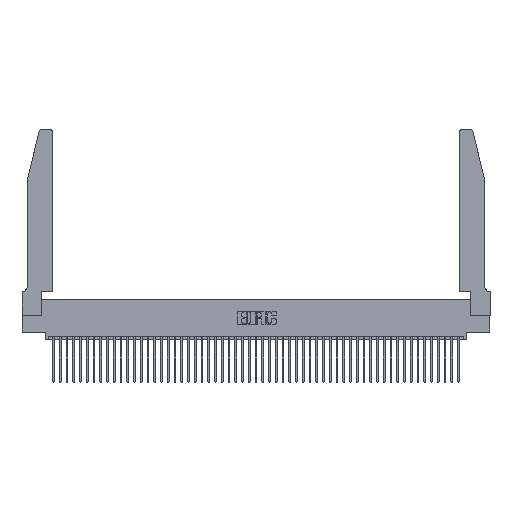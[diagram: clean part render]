
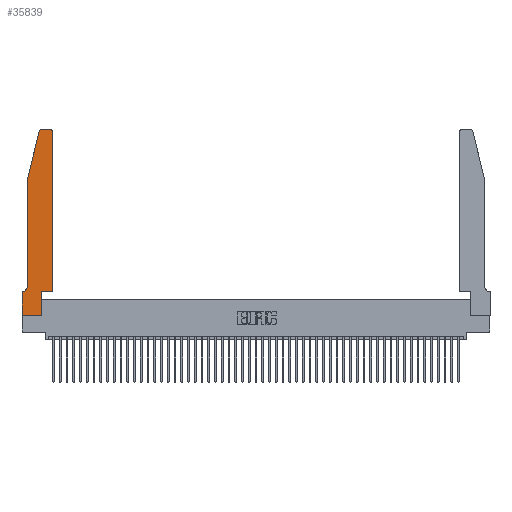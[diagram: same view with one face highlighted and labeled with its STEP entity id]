
A CAD part, top view. The second image highlights one B-rep face of the part: STEP entity #35839.
In plain terms, the highlighted planar face has unit normal (0, 0, 1).
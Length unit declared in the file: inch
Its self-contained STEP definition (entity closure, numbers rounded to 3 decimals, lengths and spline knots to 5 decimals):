
#976 = FACE_OUTER_BOUND ( 'NONE', #17542, .T. ) ;
#1077 = VERTEX_POINT ( 'NONE', #43807 ) ;
#1514 = DIRECTION ( 'NONE',  ( -1., 0., 0. ) ) ;
#1660 = DIRECTION ( 'NONE',  ( 0., 0., 1. ) ) ;
#1904 = AXIS2_PLACEMENT_3D ( 'NONE', #23242, #15806, #27826 ) ;
#1979 = ORIENTED_EDGE ( 'NONE', *, *, #27005, .T. ) ;
#2568 = VERTEX_POINT ( 'NONE', #7522 ) ;
#2646 = EDGE_CURVE ( 'NONE', #1077, #48703, #37941, .T. ) ;
#2672 = ORIENTED_EDGE ( 'NONE', *, *, #40567, .T. ) ;
#6020 = VERTEX_POINT ( 'NONE', #24661 ) ;
#7099 = VERTEX_POINT ( 'NONE', #8800 ) ;
#7431 = CARTESIAN_POINT ( 'NONE',  ( 0.0055, 0.42, 0.37 ) ) ;
#7522 = CARTESIAN_POINT ( 'NONE',  ( 0.0055, 0.35, 0.37 ) ) ;
#7527 = CARTESIAN_POINT ( 'NONE',  ( 0., 0., 0.37 ) ) ;
#7871 = VECTOR ( 'NONE', #33401, 39.37008 ) ;
#8644 = ORIENTED_EDGE ( 'NONE', *, *, #44834, .T. ) ;
#8800 = CARTESIAN_POINT ( 'NONE',  ( 0.4205, 2.75, 0.37 ) ) ;
#10366 = EDGE_CURVE ( 'NONE', #50022, #20341, #16320, .T. ) ;
#10369 = LINE ( 'NONE', #43855, #40085 ) ;
#10970 = ORIENTED_EDGE ( 'NONE', *, *, #28185, .T. ) ;
#11981 = DIRECTION ( 'NONE',  ( 1., 0., 0. ) ) ;
#12465 = CIRCLE ( 'NONE', #50095, 0.03 ) ;
#12561 = ORIENTED_EDGE ( 'NONE', *, *, #25093, .T. ) ;
#12879 = CARTESIAN_POINT ( 'NONE',  ( 0.284, 2.75, 0.37 ) ) ;
#13540 = ORIENTED_EDGE ( 'NONE', *, *, #2646, .T. ) ;
#14479 = VECTOR ( 'NONE', #48532, 39.37008 ) ;
#15806 = DIRECTION ( 'NONE',  ( 0., 0., 1. ) ) ;
#16320 = LINE ( 'NONE', #31479, #32699 ) ;
#16555 = EDGE_CURVE ( 'NONE', #7099, #48152, #25830, .T. ) ;
#16969 = CARTESIAN_POINT ( 'NONE',  ( 0.2865, 0.35, 0.37 ) ) ;
#17173 = ORIENTED_EDGE ( 'NONE', *, *, #42007, .T. ) ;
#17357 = CIRCLE ( 'NONE', #1904, 0.03 ) ;
#17542 = EDGE_LOOP ( 'NONE', ( #43510, #10970, #23034, #13540, #12561, #2672, #17173, #32982, #8644, #22302, #1979, #47942 ) ) ;
#17870 = CARTESIAN_POINT ( 'NONE',  ( 0., 0.35, 0.37 ) ) ;
#18157 = DIRECTION ( 'NONE',  ( -1., 0., 0. ) ) ;
#18282 = VERTEX_POINT ( 'NONE', #32428 ) ;
#18809 = LINE ( 'NONE', #7527, #32759 ) ;
#19646 = DIRECTION ( 'NONE',  ( 0., 0., -1. ) ) ;
#20068 = DIRECTION ( 'NONE',  ( 0., -1., 0. ) ) ;
#20341 = VERTEX_POINT ( 'NONE', #48857 ) ;
#21359 = LINE ( 'NONE', #28673, #38328 ) ;
#21648 = CARTESIAN_POINT ( 'NONE',  ( 0.0755, 0.42, 0.37 ) ) ;
#22302 = ORIENTED_EDGE ( 'NONE', *, *, #10366, .T. ) ;
#23034 = ORIENTED_EDGE ( 'NONE', *, *, #41205, .T. ) ;
#23242 = CARTESIAN_POINT ( 'NONE',  ( 0.4205, 2.72, 0.37 ) ) ;
#24175 = VERTEX_POINT ( 'NONE', #26528 ) ;
#24477 = CARTESIAN_POINT ( 'NONE',  ( 0.0755, 2., 0.37 ) ) ;
#24661 = CARTESIAN_POINT ( 'NONE',  ( 0.2865, 0., 0.37 ) ) ;
#24817 = CARTESIAN_POINT ( 'NONE',  ( 0.4505, 0.35, 0.37 ) ) ;
#25093 = EDGE_CURVE ( 'NONE', #48703, #2568, #46789, .T. ) ;
#25271 = CARTESIAN_POINT ( 'NONE',  ( 0., 0., 0.37 ) ) ;
#25412 = CARTESIAN_POINT ( 'NONE',  ( 0.284, 2.72, 0.37 ) ) ;
#25830 = LINE ( 'NONE', #37803, #33707 ) ;
#26008 = LINE ( 'NONE', #24817, #14479 ) ;
#26528 = CARTESIAN_POINT ( 'NONE',  ( 0.4505, 2.72, 0.37 ) ) ;
#26947 = DIRECTION ( 'NONE',  ( 1., 0., 0. ) ) ;
#27005 = EDGE_CURVE ( 'NONE', #20341, #24175, #26008, .T. ) ;
#27826 = DIRECTION ( 'NONE',  ( 1., 0., 0. ) ) ;
#28185 = EDGE_CURVE ( 'NONE', #48152, #28757, #12465, .T. ) ;
#28673 = CARTESIAN_POINT ( 'NONE',  ( 0.0755, 0.35, 0.37 ) ) ;
#28757 = VERTEX_POINT ( 'NONE', #44328 ) ;
#31275 = CARTESIAN_POINT ( 'NONE',  ( 0.2865, 0.35, 0.37 ) ) ;
#31479 = CARTESIAN_POINT ( 'NONE',  ( 0.4505, 0.35, 0.37 ) ) ;
#31978 = AXIS2_PLACEMENT_3D ( 'NONE', #7431, #19646, #46451 ) ;
#32428 = CARTESIAN_POINT ( 'NONE',  ( 0., 0., 0.37 ) ) ;
#32699 = VECTOR ( 'NONE', #11981, 39.37008 ) ;
#32759 = VECTOR ( 'NONE', #38567, 39.37008 ) ;
#32982 = ORIENTED_EDGE ( 'NONE', *, *, #45335, .T. ) ;
#33392 = CARTESIAN_POINT ( 'NONE',  ( 0., 0.35, 0.37 ) ) ;
#33401 = DIRECTION ( 'NONE',  ( 0., -1., 0. ) ) ;
#33404 = AXIS2_PLACEMENT_3D ( 'NONE', #33392, #49980, #26947 ) ;
#33707 = VECTOR ( 'NONE', #18157, 39.37008 ) ;
#33733 = VECTOR ( 'NONE', #20068, 39.37008 ) ;
#34818 = DIRECTION ( 'NONE',  ( 0., 1., 0. ) ) ;
#35839 = ADVANCED_FACE ( 'NONE', ( #976 ), #50145, .T. ) ;
#35868 = VECTOR ( 'NONE', #34818, 39.37008 ) ;
#37803 = CARTESIAN_POINT ( 'NONE',  ( 0.2605, 2.75, 0.37 ) ) ;
#37941 = LINE ( 'NONE', #24477, #33733 ) ;
#38328 = VECTOR ( 'NONE', #1514, 39.37008 ) ;
#38567 = DIRECTION ( 'NONE',  ( 1., 0., 0. ) ) ;
#38820 = LINE ( 'NONE', #25271, #7871 ) ;
#40085 = VECTOR ( 'NONE', #47749, 39.37008 ) ;
#40567 = EDGE_CURVE ( 'NONE', #2568, #43270, #21359, .T. ) ;
#40661 = DIRECTION ( 'NONE',  ( 1., 0., 0. ) ) ;
#41205 = EDGE_CURVE ( 'NONE', #28757, #1077, #10369, .T. ) ;
#42007 = EDGE_CURVE ( 'NONE', #43270, #18282, #38820, .T. ) ;
#43270 = VERTEX_POINT ( 'NONE', #17870 ) ;
#43510 = ORIENTED_EDGE ( 'NONE', *, *, #16555, .T. ) ;
#43807 = CARTESIAN_POINT ( 'NONE',  ( 0.0755, 2., 0.37 ) ) ;
#43855 = CARTESIAN_POINT ( 'NONE',  ( 0.0755, 2., 0.37 ) ) ;
#44328 = CARTESIAN_POINT ( 'NONE',  ( 0.25487, 2.72718, 0.37 ) ) ;
#44331 = LINE ( 'NONE', #31275, #35868 ) ;
#44834 = EDGE_CURVE ( 'NONE', #6020, #50022, #44331, .T. ) ;
#45335 = EDGE_CURVE ( 'NONE', #18282, #6020, #18809, .T. ) ;
#46451 = DIRECTION ( 'NONE',  ( -1., 0., 0. ) ) ;
#46789 = CIRCLE ( 'NONE', #31978, 0.07 ) ;
#47749 = DIRECTION ( 'NONE',  ( -0.239, -0.971, 0. ) ) ;
#47774 = EDGE_CURVE ( 'NONE', #24175, #7099, #17357, .T. ) ;
#47942 = ORIENTED_EDGE ( 'NONE', *, *, #47774, .T. ) ;
#48152 = VERTEX_POINT ( 'NONE', #12879 ) ;
#48532 = DIRECTION ( 'NONE',  ( 0., 1., 0. ) ) ;
#48703 = VERTEX_POINT ( 'NONE', #21648 ) ;
#48857 = CARTESIAN_POINT ( 'NONE',  ( 0.4505, 0.35, 0.37 ) ) ;
#49980 = DIRECTION ( 'NONE',  ( 0., 0., 1. ) ) ;
#50022 = VERTEX_POINT ( 'NONE', #16969 ) ;
#50095 = AXIS2_PLACEMENT_3D ( 'NONE', #25412, #1660, #40661 ) ;
#50145 = PLANE ( 'NONE',  #33404 ) ;
